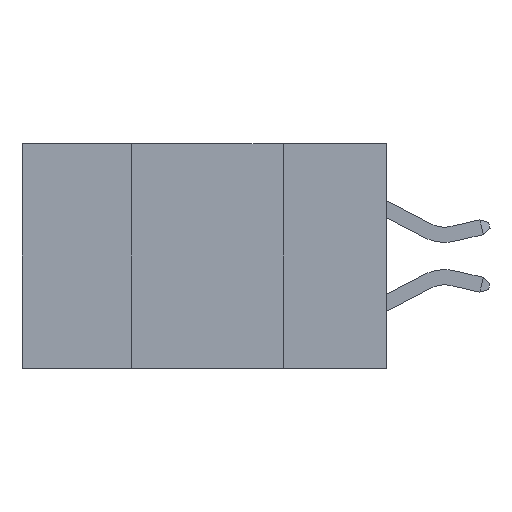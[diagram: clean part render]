
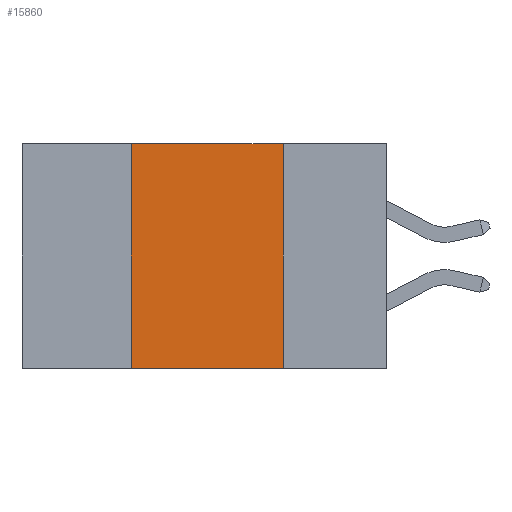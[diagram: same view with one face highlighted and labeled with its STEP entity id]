
A CAD part, left-side view. The second image highlights one B-rep face of the part: STEP entity #15860.
In plain terms, the highlighted planar face has unit normal (-1, 0, 0).
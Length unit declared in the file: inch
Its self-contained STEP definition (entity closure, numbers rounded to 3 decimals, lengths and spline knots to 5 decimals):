
#1049 = CARTESIAN_POINT ( 'NONE',  ( 0., 0.17, 0. ) ) ;
#1328 = DIRECTION ( 'NONE',  ( 0., -1., 0. ) ) ;
#2769 = DIRECTION ( 'NONE',  ( 1., 0., 0. ) ) ;
#2845 = EDGE_CURVE ( 'NONE', #15513, #9888, #10307, .T. ) ;
#2911 = VECTOR ( 'NONE', #23762, 39.37008 ) ;
#2988 = VECTOR ( 'NONE', #5784, 39.37008 ) ;
#3592 = EDGE_CURVE ( 'NONE', #11852, #6446, #8656, .T. ) ;
#4284 = EDGE_CURVE ( 'NONE', #15513, #11852, #9584, .T. ) ;
#4303 = ORIENTED_EDGE ( 'NONE', *, *, #2845, .T. ) ;
#5784 = DIRECTION ( 'NONE',  ( 0., -1., 0. ) ) ;
#6446 = VERTEX_POINT ( 'NONE', #1049 ) ;
#8222 = CARTESIAN_POINT ( 'NONE',  ( 0., 0.6, -0.37 ) ) ;
#8656 = LINE ( 'NONE', #16105, #2988 ) ;
#8998 = EDGE_LOOP ( 'NONE', ( #21460, #21492, #17225, #4303 ) ) ;
#9004 = VECTOR ( 'NONE', #1328, 39.37008 ) ;
#9228 = LINE ( 'NONE', #15690, #2911 ) ;
#9584 = LINE ( 'NONE', #10809, #19743 ) ;
#9888 = VERTEX_POINT ( 'NONE', #23596 ) ;
#9959 = EDGE_CURVE ( 'NONE', #6446, #9888, #9228, .T. ) ;
#10307 = LINE ( 'NONE', #8222, #9004 ) ;
#10638 = DIRECTION ( 'NONE',  ( 0., 0., 1. ) ) ;
#10809 = CARTESIAN_POINT ( 'NONE',  ( 0., 0.42, 0. ) ) ;
#11852 = VERTEX_POINT ( 'NONE', #25569 ) ;
#13211 = PLANE ( 'NONE',  #16577 ) ;
#15246 = CARTESIAN_POINT ( 'NONE',  ( 0., 0.6, 0. ) ) ;
#15513 = VERTEX_POINT ( 'NONE', #18246 ) ;
#15690 = CARTESIAN_POINT ( 'NONE',  ( 0., 0.17, 0. ) ) ;
#15860 = ADVANCED_FACE ( 'NONE', ( #18892 ), #13211, .F. ) ;
#16105 = CARTESIAN_POINT ( 'NONE',  ( 0., 0.6, 0. ) ) ;
#16577 = AXIS2_PLACEMENT_3D ( 'NONE', #15246, #2769, #17285 ) ;
#17225 = ORIENTED_EDGE ( 'NONE', *, *, #4284, .F. ) ;
#17285 = DIRECTION ( 'NONE',  ( 0., 0., -1. ) ) ;
#18246 = CARTESIAN_POINT ( 'NONE',  ( 0., 0.42, -0.37 ) ) ;
#18892 = FACE_OUTER_BOUND ( 'NONE', #8998, .T. ) ;
#19743 = VECTOR ( 'NONE', #10638, 39.37008 ) ;
#21460 = ORIENTED_EDGE ( 'NONE', *, *, #9959, .F. ) ;
#21492 = ORIENTED_EDGE ( 'NONE', *, *, #3592, .F. ) ;
#23596 = CARTESIAN_POINT ( 'NONE',  ( 0., 0.17, -0.37 ) ) ;
#23762 = DIRECTION ( 'NONE',  ( 0., 0., -1. ) ) ;
#25569 = CARTESIAN_POINT ( 'NONE',  ( 0., 0.42, 0. ) ) ;
